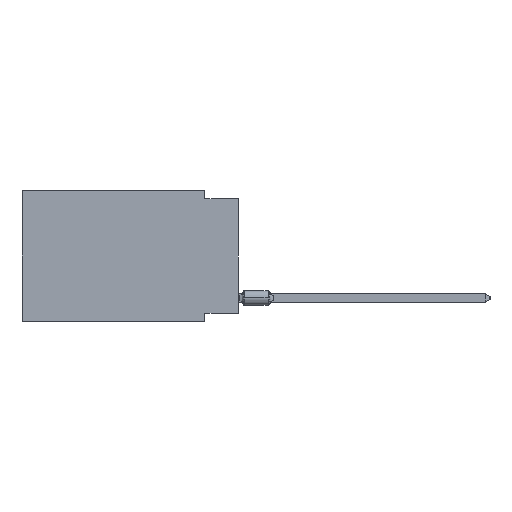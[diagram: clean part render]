
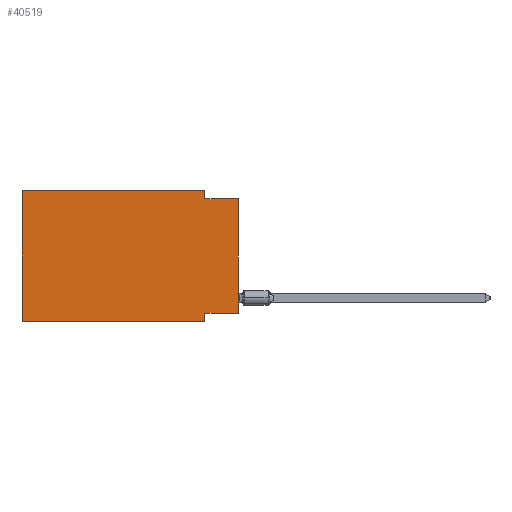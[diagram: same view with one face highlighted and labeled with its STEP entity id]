
A CAD part, left-side view. The second image highlights one B-rep face of the part: STEP entity #40519.
In plain terms, the highlighted planar face has unit normal (-1, 0, 0).
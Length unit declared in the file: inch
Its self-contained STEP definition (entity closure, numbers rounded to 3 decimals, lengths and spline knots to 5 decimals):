
#1143 = CARTESIAN_POINT ( 'NONE',  ( 0., 0.1, 0. ) ) ;
#1475 = ORIENTED_EDGE ( 'NONE', *, *, #68839, .F. ) ;
#1916 = CARTESIAN_POINT ( 'NONE',  ( 0., 0.1, -0.39 ) ) ;
#2714 = ORIENTED_EDGE ( 'NONE', *, *, #81109, .F. ) ;
#3102 = FACE_OUTER_BOUND ( 'NONE', #36092, .T. ) ;
#3178 = DIRECTION ( 'NONE',  ( 0., -1., 0. ) ) ;
#8907 = VERTEX_POINT ( 'NONE', #30563 ) ;
#9272 = VECTOR ( 'NONE', #10253, 39.37008 ) ;
#9453 = LINE ( 'NONE', #34915, #31370 ) ;
#10253 = DIRECTION ( 'NONE',  ( 0., 0., -1. ) ) ;
#14437 = VERTEX_POINT ( 'NONE', #1143 ) ;
#15523 = VERTEX_POINT ( 'NONE', #52891 ) ;
#19528 = CARTESIAN_POINT ( 'NONE',  ( 0., 0., -0.365 ) ) ;
#19730 = CARTESIAN_POINT ( 'NONE',  ( 0., 0.1, -0.025 ) ) ;
#20684 = CARTESIAN_POINT ( 'NONE',  ( 0., 0., -0.025 ) ) ;
#21129 = ORIENTED_EDGE ( 'NONE', *, *, #72848, .F. ) ;
#21509 = AXIS2_PLACEMENT_3D ( 'NONE', #41543, #54048, #67027 ) ;
#22308 = ORIENTED_EDGE ( 'NONE', *, *, #72736, .T. ) ;
#22709 = VECTOR ( 'NONE', #37789, 39.37008 ) ;
#24809 = CARTESIAN_POINT ( 'NONE',  ( 0., 0.645, 0. ) ) ;
#28575 = PLANE ( 'NONE',  #21509 ) ;
#30563 = CARTESIAN_POINT ( 'NONE',  ( 0., 0.645, -0.39 ) ) ;
#31115 = CARTESIAN_POINT ( 'NONE',  ( 0., 0., 0. ) ) ;
#31149 = ORIENTED_EDGE ( 'NONE', *, *, #34769, .F. ) ;
#31370 = VECTOR ( 'NONE', #3178, 39.37008 ) ;
#33879 = ORIENTED_EDGE ( 'NONE', *, *, #39148, .T. ) ;
#34769 = EDGE_CURVE ( 'NONE', #50191, #60650, #42341, .T. ) ;
#34915 = CARTESIAN_POINT ( 'NONE',  ( 0., 0.645, -0.39 ) ) ;
#36092 = EDGE_LOOP ( 'NONE', ( #33879, #74686, #42439, #1475, #21129, #22308, #2714, #31149 ) ) ;
#36169 = CARTESIAN_POINT ( 'NONE',  ( 0., 0.645, 0. ) ) ;
#37789 = DIRECTION ( 'NONE',  ( 0., 0., 1. ) ) ;
#38909 = CARTESIAN_POINT ( 'NONE',  ( 0., 0.1, -0.365 ) ) ;
#39148 = EDGE_CURVE ( 'NONE', #50191, #15523, #76644, .T. ) ;
#39224 = VECTOR ( 'NONE', #51196, 39.37008 ) ;
#40519 = ADVANCED_FACE ( 'NONE', ( #3102 ), #28575, .F. ) ;
#41543 = CARTESIAN_POINT ( 'NONE',  ( 0., 0.645, 0. ) ) ;
#41904 = VERTEX_POINT ( 'NONE', #19730 ) ;
#42341 = LINE ( 'NONE', #80377, #67780 ) ;
#42439 = ORIENTED_EDGE ( 'NONE', *, *, #81390, .F. ) ;
#43245 = LINE ( 'NONE', #62867, #58029 ) ;
#49893 = DIRECTION ( 'NONE',  ( 0., 0., 1. ) ) ;
#50191 = VERTEX_POINT ( 'NONE', #19528 ) ;
#50664 = VERTEX_POINT ( 'NONE', #1916 ) ;
#51196 = DIRECTION ( 'NONE',  ( 0., -1., 0. ) ) ;
#52891 = CARTESIAN_POINT ( 'NONE',  ( 0., 0., -0.025 ) ) ;
#53014 = LINE ( 'NONE', #68388, #63992 ) ;
#54048 = DIRECTION ( 'NONE',  ( 1., 0., 0. ) ) ;
#58029 = VECTOR ( 'NONE', #49893, 39.37008 ) ;
#58904 = VECTOR ( 'NONE', #82108, 39.37008 ) ;
#58943 = VERTEX_POINT ( 'NONE', #24809 ) ;
#59557 = CARTESIAN_POINT ( 'NONE',  ( 0., 0.1, -0.39 ) ) ;
#60650 = VERTEX_POINT ( 'NONE', #38909 ) ;
#62109 = DIRECTION ( 'NONE',  ( 0., 0., -1. ) ) ;
#62867 = CARTESIAN_POINT ( 'NONE',  ( 0., 0.645, 0. ) ) ;
#63992 = VECTOR ( 'NONE', #62109, 39.37008 ) ;
#67027 = DIRECTION ( 'NONE',  ( 0., 0., -1. ) ) ;
#67780 = VECTOR ( 'NONE', #69043, 39.37008 ) ;
#67934 = LINE ( 'NONE', #36169, #58904 ) ;
#68388 = CARTESIAN_POINT ( 'NONE',  ( 0., 0.1, 0. ) ) ;
#68839 = EDGE_CURVE ( 'NONE', #58943, #14437, #67934, .T. ) ;
#69043 = DIRECTION ( 'NONE',  ( 0., 1., 0. ) ) ;
#71273 = EDGE_CURVE ( 'NONE', #41904, #15523, #71679, .T. ) ;
#71679 = LINE ( 'NONE', #20684, #39224 ) ;
#72736 = EDGE_CURVE ( 'NONE', #8907, #50664, #9453, .T. ) ;
#72848 = EDGE_CURVE ( 'NONE', #8907, #58943, #43245, .T. ) ;
#73777 = LINE ( 'NONE', #59557, #9272 ) ;
#74686 = ORIENTED_EDGE ( 'NONE', *, *, #71273, .F. ) ;
#76644 = LINE ( 'NONE', #31115, #22709 ) ;
#80377 = CARTESIAN_POINT ( 'NONE',  ( 0., 0., -0.365 ) ) ;
#81109 = EDGE_CURVE ( 'NONE', #60650, #50664, #73777, .T. ) ;
#81390 = EDGE_CURVE ( 'NONE', #14437, #41904, #53014, .T. ) ;
#82108 = DIRECTION ( 'NONE',  ( 0., -1., 0. ) ) ;
